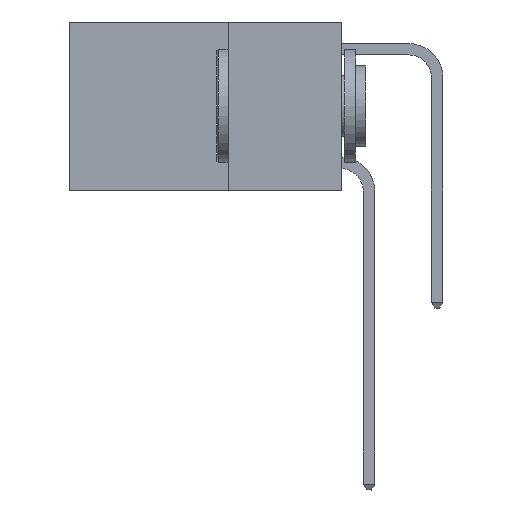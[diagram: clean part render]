
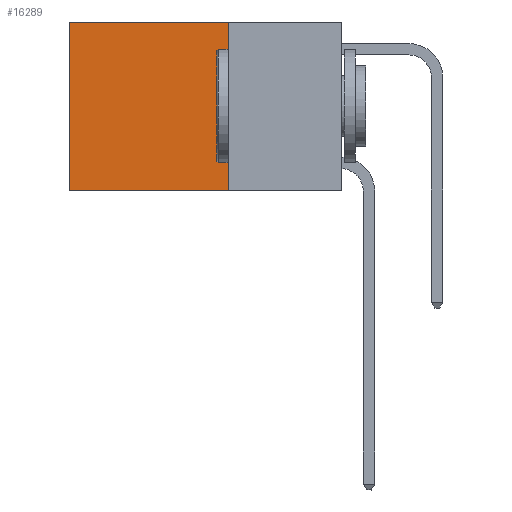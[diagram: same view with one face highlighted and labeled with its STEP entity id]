
A CAD part, left-side view. The second image highlights one B-rep face of the part: STEP entity #16289.
In plain terms, the highlighted planar face has unit normal (-1, 0, 0).
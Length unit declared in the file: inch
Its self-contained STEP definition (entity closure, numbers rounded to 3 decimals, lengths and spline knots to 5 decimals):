
#284 = VECTOR ( 'NONE', #17054, 39.37008 ) ;
#1409 = VERTEX_POINT ( 'NONE', #3062 ) ;
#1768 = DIRECTION ( 'NONE',  ( 1., 0., 0. ) ) ;
#2438 = VERTEX_POINT ( 'NONE', #11749 ) ;
#2448 = VECTOR ( 'NONE', #20502, 39.37008 ) ;
#2725 = CARTESIAN_POINT ( 'NONE',  ( 0.2625, 0.25, 0. ) ) ;
#3009 = VECTOR ( 'NONE', #15959, 39.37008 ) ;
#3062 = CARTESIAN_POINT ( 'NONE',  ( 0.2625, 0.6, -0.37 ) ) ;
#3713 = VERTEX_POINT ( 'NONE', #22576 ) ;
#4893 = CARTESIAN_POINT ( 'NONE',  ( 0.2625, 0.25, 0. ) ) ;
#6937 = VECTOR ( 'NONE', #20727, 39.37008 ) ;
#7539 = LINE ( 'NONE', #7973, #6937 ) ;
#7721 = CARTESIAN_POINT ( 'NONE',  ( 0.2625, 0.25, 0. ) ) ;
#7973 = CARTESIAN_POINT ( 'NONE',  ( 0.2625, 0.25, -0.37 ) ) ;
#8479 = EDGE_CURVE ( 'NONE', #3713, #1409, #7539, .T. ) ;
#10433 = ORIENTED_EDGE ( 'NONE', *, *, #22959, .T. ) ;
#11060 = VERTEX_POINT ( 'NONE', #2725 ) ;
#11749 = CARTESIAN_POINT ( 'NONE',  ( 0.2625, 0.6, 0. ) ) ;
#11950 = ORIENTED_EDGE ( 'NONE', *, *, #14507, .F. ) ;
#12910 = PLANE ( 'NONE',  #19215 ) ;
#13383 = ORIENTED_EDGE ( 'NONE', *, *, #16109, .T. ) ;
#13478 = CARTESIAN_POINT ( 'NONE',  ( 0.2625, 0.6, 0. ) ) ;
#14507 = EDGE_CURVE ( 'NONE', #11060, #3713, #17240, .T. ) ;
#14755 = DIRECTION ( 'NONE',  ( 0., 0., -1. ) ) ;
#15077 = LINE ( 'NONE', #13478, #284 ) ;
#15959 = DIRECTION ( 'NONE',  ( 0., 1., 0. ) ) ;
#16109 = EDGE_CURVE ( 'NONE', #11060, #2438, #16614, .T. ) ;
#16289 = ADVANCED_FACE ( 'NONE', ( #22193 ), #12910, .F. ) ;
#16614 = LINE ( 'NONE', #4893, #3009 ) ;
#17054 = DIRECTION ( 'NONE',  ( 0., 0., -1. ) ) ;
#17240 = LINE ( 'NONE', #7721, #2448 ) ;
#19215 = AXIS2_PLACEMENT_3D ( 'NONE', #20062, #1768, #14755 ) ;
#19273 = ORIENTED_EDGE ( 'NONE', *, *, #8479, .F. ) ;
#20062 = CARTESIAN_POINT ( 'NONE',  ( 0.2625, 0.25, 0. ) ) ;
#20502 = DIRECTION ( 'NONE',  ( 0., 0., -1. ) ) ;
#20727 = DIRECTION ( 'NONE',  ( 0., 1., 0. ) ) ;
#22193 = FACE_OUTER_BOUND ( 'NONE', #22328, .T. ) ;
#22328 = EDGE_LOOP ( 'NONE', ( #10433, #19273, #11950, #13383 ) ) ;
#22576 = CARTESIAN_POINT ( 'NONE',  ( 0.2625, 0.25, -0.37 ) ) ;
#22959 = EDGE_CURVE ( 'NONE', #2438, #1409, #15077, .T. ) ;
